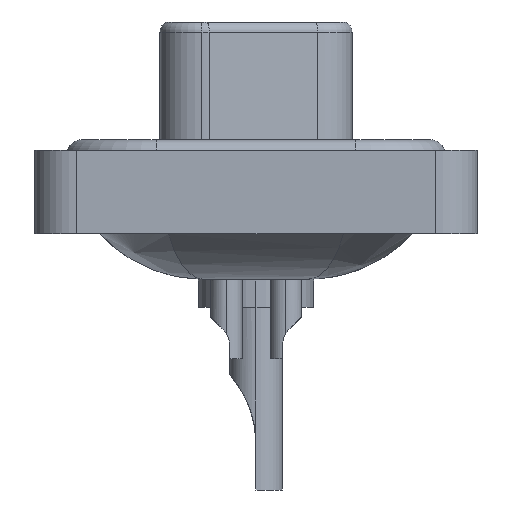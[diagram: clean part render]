
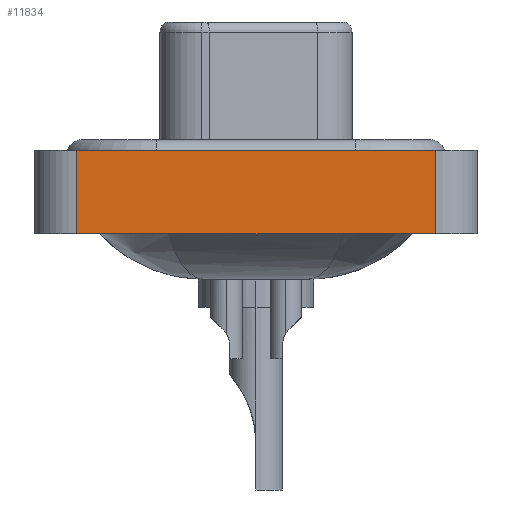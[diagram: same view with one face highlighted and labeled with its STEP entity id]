
A CAD part, left-side view. The second image highlights one B-rep face of the part: STEP entity #11834.
In plain terms, the highlighted planar face has unit normal (-1, 0, 0).
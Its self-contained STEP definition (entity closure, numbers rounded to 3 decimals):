
#85 = VERTEX_POINT ( 'NONE', #20501 ) ;
#237 = VERTEX_POINT ( 'NONE', #11235 ) ;
#1364 = ORIENTED_EDGE ( 'NONE', *, *, #15048, .F. ) ;
#2086 = LINE ( 'NONE', #13637, #3648 ) ;
#2389 = CARTESIAN_POINT ( 'NONE',  ( -7.3, -8.55, 0.4 ) ) ;
#2770 = EDGE_CURVE ( 'NONE', #237, #19847, #2086, .T. ) ;
#3203 = VECTOR ( 'NONE', #19240, 1000. ) ;
#3387 = DIRECTION ( 'NONE',  ( 0., 0., 1. ) ) ;
#3648 = VECTOR ( 'NONE', #3387, 1000. ) ;
#4358 = DIRECTION ( 'NONE',  ( 0., -1., 0. ) ) ;
#5840 = DIRECTION ( 'NONE',  ( 0., -1., 0. ) ) ;
#6304 = EDGE_LOOP ( 'NONE', ( #18252, #19281, #1364, #9283 ) ) ;
#8504 = FACE_OUTER_BOUND ( 'NONE', #6304, .T. ) ;
#9283 = ORIENTED_EDGE ( 'NONE', *, *, #17865, .T. ) ;
#9556 = VECTOR ( 'NONE', #5840, 1000. ) ;
#10269 = VECTOR ( 'NONE', #4358, 1000. ) ;
#11235 = CARTESIAN_POINT ( 'NONE',  ( -7.3, -8.55, -3.6 ) ) ;
#11834 = ADVANCED_FACE ( 'NONE', ( #8504 ), #21058, .T. ) ;
#12591 = CARTESIAN_POINT ( 'NONE',  ( -7.3, -8.55, -3.6 ) ) ;
#12791 = DIRECTION ( 'NONE',  ( -1., 0., 0. ) ) ;
#12900 = CARTESIAN_POINT ( 'NONE',  ( -7.3, -8.55, -3.6 ) ) ;
#13637 = CARTESIAN_POINT ( 'NONE',  ( -7.3, -8.55, -3.6 ) ) ;
#14136 = CARTESIAN_POINT ( 'NONE',  ( -7.3, -8.55, 0.4 ) ) ;
#14289 = LINE ( 'NONE', #20850, #3203 ) ;
#15048 = EDGE_CURVE ( 'NONE', #85, #19789, #14289, .T. ) ;
#15545 = LINE ( 'NONE', #2389, #9556 ) ;
#17596 = AXIS2_PLACEMENT_3D ( 'NONE', #12900, #12791, #19459 ) ;
#17865 = EDGE_CURVE ( 'NONE', #85, #237, #20749, .T. ) ;
#18094 = EDGE_CURVE ( 'NONE', #19789, #19847, #15545, .T. ) ;
#18252 = ORIENTED_EDGE ( 'NONE', *, *, #2770, .T. ) ;
#19240 = DIRECTION ( 'NONE',  ( 0., 0., 1. ) ) ;
#19281 = ORIENTED_EDGE ( 'NONE', *, *, #18094, .F. ) ;
#19459 = DIRECTION ( 'NONE',  ( 0., 0., 1. ) ) ;
#19789 = VERTEX_POINT ( 'NONE', #19942 ) ;
#19847 = VERTEX_POINT ( 'NONE', #14136 ) ;
#19942 = CARTESIAN_POINT ( 'NONE',  ( -7.3, 8.55, 0.4 ) ) ;
#20501 = CARTESIAN_POINT ( 'NONE',  ( -7.3, 8.55, -3.6 ) ) ;
#20749 = LINE ( 'NONE', #12591, #10269 ) ;
#20850 = CARTESIAN_POINT ( 'NONE',  ( -7.3, 8.55, -3.6 ) ) ;
#21058 = PLANE ( 'NONE',  #17596 ) ;
